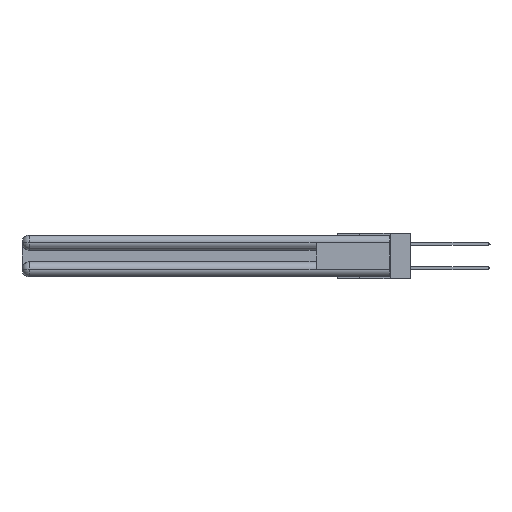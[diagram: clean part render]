
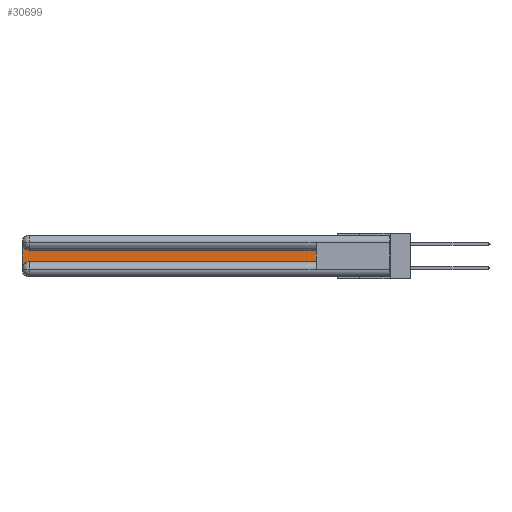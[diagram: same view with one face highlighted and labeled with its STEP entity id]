
A CAD part, left-side view. The second image highlights one B-rep face of the part: STEP entity #30699.
In plain terms, the highlighted planar face has unit normal (-1, 0, 0).
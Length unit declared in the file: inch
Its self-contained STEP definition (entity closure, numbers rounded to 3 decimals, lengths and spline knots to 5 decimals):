
#477 = CARTESIAN_POINT ( 'NONE',  ( 0.075, 0.6, -0.1225 ) ) ;
#519 = VERTEX_POINT ( 'NONE', #17002 ) ;
#2059 = LINE ( 'NONE', #21915, #8592 ) ;
#2145 = VERTEX_POINT ( 'NONE', #25928 ) ;
#2586 = CARTESIAN_POINT ( 'NONE',  ( 0.075, 0.6, -0.2175 ) ) ;
#3625 = CARTESIAN_POINT ( 'NONE',  ( 0.075, 2.94, -0.0625 ) ) ;
#4084 = DIRECTION ( 'NONE',  ( 0., -1., 0. ) ) ;
#4171 = LINE ( 'NONE', #6407, #16387 ) ;
#4744 = LINE ( 'NONE', #477, #24818 ) ;
#5796 = VERTEX_POINT ( 'NONE', #10016 ) ;
#6028 = DIRECTION ( 'NONE',  ( 0., 0., -1. ) ) ;
#6146 = PLANE ( 'NONE',  #33527 ) ;
#6407 = CARTESIAN_POINT ( 'NONE',  ( 0.075, 3., -0.2175 ) ) ;
#6797 = CARTESIAN_POINT ( 'NONE',  ( 0.075, 0.6, -0.2175 ) ) ;
#7666 = ORIENTED_EDGE ( 'NONE', *, *, #17368, .T. ) ;
#8592 = VECTOR ( 'NONE', #35663, 39.37008 ) ;
#9486 = CARTESIAN_POINT ( 'NONE',  ( 0.075, 3., -0.0625 ) ) ;
#9541 = DIRECTION ( 'NONE',  ( 1., 0., 0. ) ) ;
#10016 = CARTESIAN_POINT ( 'NONE',  ( 0.075, 2.94, -0.2175 ) ) ;
#10968 = VECTOR ( 'NONE', #4084, 39.37008 ) ;
#11543 = ORIENTED_EDGE ( 'NONE', *, *, #31746, .T. ) ;
#14210 = AXIS2_PLACEMENT_3D ( 'NONE', #15482, #9541, #18157 ) ;
#14540 = EDGE_LOOP ( 'NONE', ( #22039, #7666, #19019, #32460, #11543, #26595 ) ) ;
#15482 = CARTESIAN_POINT ( 'NONE',  ( 0.075, 2.94, -0.2775 ) ) ;
#16387 = VECTOR ( 'NONE', #34159, 39.37008 ) ;
#16965 = CARTESIAN_POINT ( 'NONE',  ( 0.075, 3., -0.1225 ) ) ;
#17002 = CARTESIAN_POINT ( 'NONE',  ( 0.075, 2.94, -0.1225 ) ) ;
#17152 = VERTEX_POINT ( 'NONE', #2586 ) ;
#17368 = EDGE_CURVE ( 'NONE', #519, #26404, #21838, .T. ) ;
#18157 = DIRECTION ( 'NONE',  ( 0., 0., -1. ) ) ;
#19019 = ORIENTED_EDGE ( 'NONE', *, *, #23166, .T. ) ;
#19061 = VERTEX_POINT ( 'NONE', #32289 ) ;
#19892 = DIRECTION ( 'NONE',  ( 1., 0., 0. ) ) ;
#21292 = EDGE_CURVE ( 'NONE', #19061, #519, #4744, .T. ) ;
#21838 = CIRCLE ( 'NONE', #29279, 0.06 ) ;
#21915 = CARTESIAN_POINT ( 'NONE',  ( 0.075, 0.6, -0.2175 ) ) ;
#22039 = ORIENTED_EDGE ( 'NONE', *, *, #21292, .T. ) ;
#23072 = DIRECTION ( 'NONE',  ( 0., 1., 0. ) ) ;
#23166 = EDGE_CURVE ( 'NONE', #26404, #2145, #4171, .T. ) ;
#23485 = DIRECTION ( 'NONE',  ( 0., 0., -1. ) ) ;
#24818 = VECTOR ( 'NONE', #23072, 39.37008 ) ;
#25928 = CARTESIAN_POINT ( 'NONE',  ( 0.075, 3., -0.2775 ) ) ;
#25944 = DIRECTION ( 'NONE',  ( 1., 0., 0. ) ) ;
#26404 = VERTEX_POINT ( 'NONE', #9486 ) ;
#26595 = ORIENTED_EDGE ( 'NONE', *, *, #28984, .T. ) ;
#26749 = FACE_OUTER_BOUND ( 'NONE', #14540, .T. ) ;
#28984 = EDGE_CURVE ( 'NONE', #17152, #19061, #2059, .T. ) ;
#29279 = AXIS2_PLACEMENT_3D ( 'NONE', #3625, #25944, #23485 ) ;
#30699 = ADVANCED_FACE ( 'NONE', ( #26749 ), #6146, .F. ) ;
#31746 = EDGE_CURVE ( 'NONE', #5796, #17152, #34035, .T. ) ;
#32289 = CARTESIAN_POINT ( 'NONE',  ( 0.075, 0.6, -0.1225 ) ) ;
#32460 = ORIENTED_EDGE ( 'NONE', *, *, #34842, .T. ) ;
#33527 = AXIS2_PLACEMENT_3D ( 'NONE', #16965, #19892, #6028 ) ;
#34035 = LINE ( 'NONE', #6797, #10968 ) ;
#34159 = DIRECTION ( 'NONE',  ( 0., 0., -1. ) ) ;
#34178 = CIRCLE ( 'NONE', #14210, 0.06 ) ;
#34842 = EDGE_CURVE ( 'NONE', #2145, #5796, #34178, .T. ) ;
#35663 = DIRECTION ( 'NONE',  ( 0., 0., 1. ) ) ;
